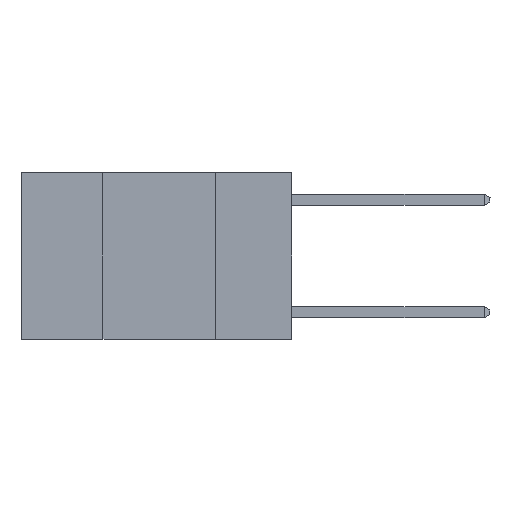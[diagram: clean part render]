
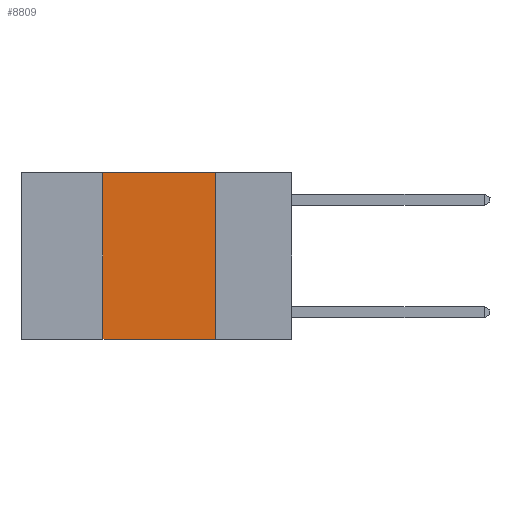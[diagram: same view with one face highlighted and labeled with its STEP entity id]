
A CAD part, left-side view. The second image highlights one B-rep face of the part: STEP entity #8809.
In plain terms, the highlighted planar face has unit normal (-1, 0, 0).
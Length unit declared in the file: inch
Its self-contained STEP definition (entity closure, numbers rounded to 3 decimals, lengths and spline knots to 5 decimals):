
#499 = LINE ( 'NONE', #4652, #10655 ) ;
#1089 = DIRECTION ( 'NONE',  ( 0., 0., -1. ) ) ;
#1285 = DIRECTION ( 'NONE',  ( 0., -1., 0. ) ) ;
#1335 = CARTESIAN_POINT ( 'NONE',  ( 0., 0.42, 0. ) ) ;
#1465 = DIRECTION ( 'NONE',  ( 0., 0., 1. ) ) ;
#1475 = CARTESIAN_POINT ( 'NONE',  ( 0., 0.42, -0.37 ) ) ;
#2150 = DIRECTION ( 'NONE',  ( 1., 0., 0. ) ) ;
#2707 = EDGE_CURVE ( 'NONE', #10343, #6414, #499, .T. ) ;
#3640 = LINE ( 'NONE', #7560, #6719 ) ;
#4652 = CARTESIAN_POINT ( 'NONE',  ( 0., 0.6, 0. ) ) ;
#5018 = VERTEX_POINT ( 'NONE', #1475 ) ;
#5020 = FACE_OUTER_BOUND ( 'NONE', #6447, .T. ) ;
#5491 = LINE ( 'NONE', #9662, #7219 ) ;
#6044 = CARTESIAN_POINT ( 'NONE',  ( 0., 0.17, 0. ) ) ;
#6188 = CARTESIAN_POINT ( 'NONE',  ( 0., 0.17, -0.37 ) ) ;
#6414 = VERTEX_POINT ( 'NONE', #6044 ) ;
#6447 = EDGE_LOOP ( 'NONE', ( #9399, #11261, #12108, #11391 ) ) ;
#6719 = VECTOR ( 'NONE', #1285, 39.37008 ) ;
#7219 = VECTOR ( 'NONE', #1465, 39.37008 ) ;
#7279 = PLANE ( 'NONE',  #13247 ) ;
#7500 = LINE ( 'NONE', #12253, #8729 ) ;
#7560 = CARTESIAN_POINT ( 'NONE',  ( 0., 0.6, -0.37 ) ) ;
#8147 = DIRECTION ( 'NONE',  ( 0., 0., -1. ) ) ;
#8729 = VECTOR ( 'NONE', #1089, 39.37008 ) ;
#8809 = ADVANCED_FACE ( 'NONE', ( #5020 ), #7279, .F. ) ;
#9399 = ORIENTED_EDGE ( 'NONE', *, *, #13231, .F. ) ;
#9662 = CARTESIAN_POINT ( 'NONE',  ( 0., 0.42, 0. ) ) ;
#9829 = EDGE_CURVE ( 'NONE', #5018, #10167, #3640, .T. ) ;
#10167 = VERTEX_POINT ( 'NONE', #6188 ) ;
#10343 = VERTEX_POINT ( 'NONE', #1335 ) ;
#10655 = VECTOR ( 'NONE', #12741, 39.37008 ) ;
#11261 = ORIENTED_EDGE ( 'NONE', *, *, #2707, .F. ) ;
#11391 = ORIENTED_EDGE ( 'NONE', *, *, #9829, .T. ) ;
#12108 = ORIENTED_EDGE ( 'NONE', *, *, #12618, .F. ) ;
#12253 = CARTESIAN_POINT ( 'NONE',  ( 0., 0.17, 0. ) ) ;
#12613 = CARTESIAN_POINT ( 'NONE',  ( 0., 0.6, 0. ) ) ;
#12618 = EDGE_CURVE ( 'NONE', #5018, #10343, #5491, .T. ) ;
#12741 = DIRECTION ( 'NONE',  ( 0., -1., 0. ) ) ;
#13231 = EDGE_CURVE ( 'NONE', #6414, #10167, #7500, .T. ) ;
#13247 = AXIS2_PLACEMENT_3D ( 'NONE', #12613, #2150, #8147 ) ;
